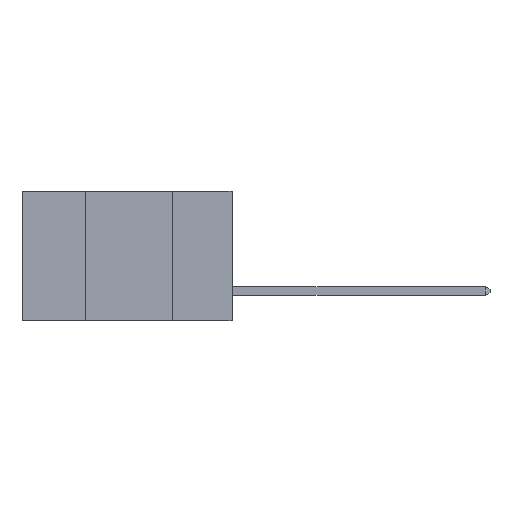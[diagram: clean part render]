
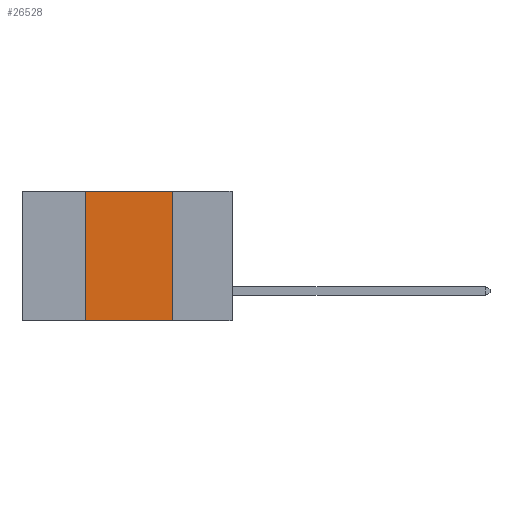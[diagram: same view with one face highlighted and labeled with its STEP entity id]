
A CAD part, left-side view. The second image highlights one B-rep face of the part: STEP entity #26528.
In plain terms, the highlighted planar face has unit normal (-1, 0, 0).
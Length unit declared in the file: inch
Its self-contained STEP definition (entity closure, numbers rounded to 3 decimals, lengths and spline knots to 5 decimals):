
#1016 = CARTESIAN_POINT ( 'NONE',  ( 0., 0.17, 0. ) ) ;
#1438 = EDGE_CURVE ( 'NONE', #6374, #11883, #30267, .T. ) ;
#2103 = LINE ( 'NONE', #1016, #27902 ) ;
#4378 = AXIS2_PLACEMENT_3D ( 'NONE', #7469, #27313, #12557 ) ;
#4481 = EDGE_CURVE ( 'NONE', #6374, #4699, #26926, .T. ) ;
#4699 = VERTEX_POINT ( 'NONE', #31784 ) ;
#5178 = ORIENTED_EDGE ( 'NONE', *, *, #23731, .F. ) ;
#6328 = EDGE_CURVE ( 'NONE', #11883, #10472, #31006, .T. ) ;
#6374 = VERTEX_POINT ( 'NONE', #23961 ) ;
#7406 = CARTESIAN_POINT ( 'NONE',  ( 0., 0.17, 0. ) ) ;
#7469 = CARTESIAN_POINT ( 'NONE',  ( 0., 0.6, 0. ) ) ;
#8823 = DIRECTION ( 'NONE',  ( 0., 0., -1. ) ) ;
#10062 = PLANE ( 'NONE',  #4378 ) ;
#10332 = CARTESIAN_POINT ( 'NONE',  ( 0., 0.42, 0. ) ) ;
#10472 = VERTEX_POINT ( 'NONE', #7406 ) ;
#11367 = CARTESIAN_POINT ( 'NONE',  ( 0., 0.6, -0.37 ) ) ;
#11377 = CARTESIAN_POINT ( 'NONE',  ( 0., 0.6, 0. ) ) ;
#11561 = CARTESIAN_POINT ( 'NONE',  ( 0., 0.42, 0. ) ) ;
#11883 = VERTEX_POINT ( 'NONE', #11561 ) ;
#12557 = DIRECTION ( 'NONE',  ( 0., 0., -1. ) ) ;
#21634 = EDGE_LOOP ( 'NONE', ( #5178, #25800, #32033, #30075 ) ) ;
#22171 = FACE_OUTER_BOUND ( 'NONE', #21634, .T. ) ;
#23731 = EDGE_CURVE ( 'NONE', #10472, #4699, #2103, .T. ) ;
#23961 = CARTESIAN_POINT ( 'NONE',  ( 0., 0.42, -0.37 ) ) ;
#24451 = VECTOR ( 'NONE', #31063, 39.37008 ) ;
#25800 = ORIENTED_EDGE ( 'NONE', *, *, #6328, .F. ) ;
#26128 = DIRECTION ( 'NONE',  ( 0., -1., 0. ) ) ;
#26150 = VECTOR ( 'NONE', #26128, 39.37008 ) ;
#26528 = ADVANCED_FACE ( 'NONE', ( #22171 ), #10062, .F. ) ;
#26926 = LINE ( 'NONE', #11367, #26150 ) ;
#27313 = DIRECTION ( 'NONE',  ( 1., 0., 0. ) ) ;
#27902 = VECTOR ( 'NONE', #8823, 39.37008 ) ;
#29496 = VECTOR ( 'NONE', #29829, 39.37008 ) ;
#29829 = DIRECTION ( 'NONE',  ( 0., 0., 1. ) ) ;
#30075 = ORIENTED_EDGE ( 'NONE', *, *, #4481, .T. ) ;
#30267 = LINE ( 'NONE', #10332, #29496 ) ;
#31006 = LINE ( 'NONE', #11377, #24451 ) ;
#31063 = DIRECTION ( 'NONE',  ( 0., -1., 0. ) ) ;
#31784 = CARTESIAN_POINT ( 'NONE',  ( 0., 0.17, -0.37 ) ) ;
#32033 = ORIENTED_EDGE ( 'NONE', *, *, #1438, .F. ) ;
